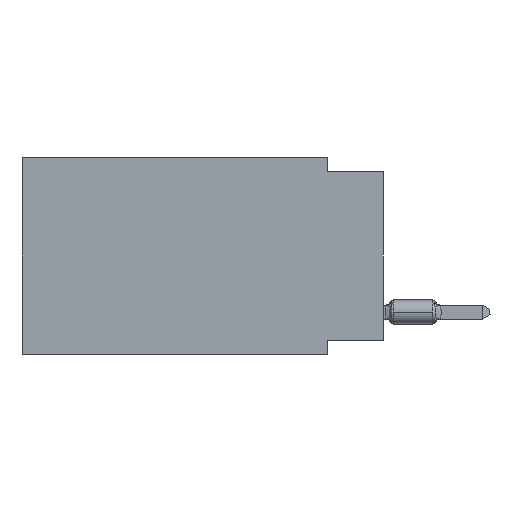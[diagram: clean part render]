
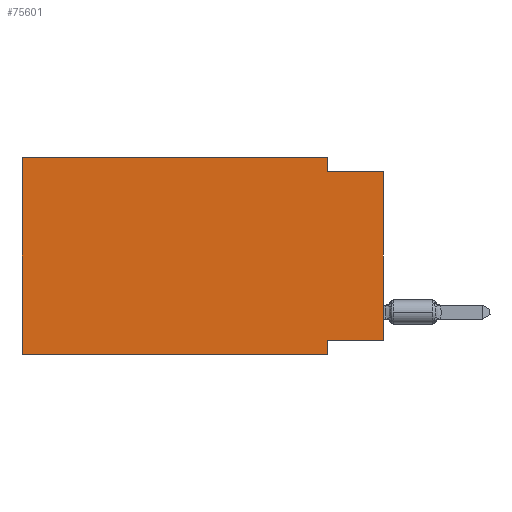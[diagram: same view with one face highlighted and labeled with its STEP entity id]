
A CAD part, left-side view. The second image highlights one B-rep face of the part: STEP entity #75601.
In plain terms, the highlighted planar face has unit normal (-1, 0, 0).
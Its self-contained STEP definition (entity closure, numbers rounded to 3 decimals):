
#530 = ORIENTED_EDGE ( 'NONE', *, *, #30145, .F. ) ;
#907 = DIRECTION ( 'NONE',  ( 1., 0., 0. ) ) ;
#2141 = VERTEX_POINT ( 'NONE', #28558 ) ;
#4248 = EDGE_CURVE ( 'NONE', #70597, #76790, #23157, .T. ) ;
#8941 = DIRECTION ( 'NONE',  ( 0., 0., -1. ) ) ;
#9344 = VECTOR ( 'NONE', #46747, 1000. ) ;
#9531 = DIRECTION ( 'NONE',  ( 0., -1., 0. ) ) ;
#12364 = CARTESIAN_POINT ( 'NONE',  ( 0., 2.54, 0. ) ) ;
#13084 = VECTOR ( 'NONE', #8941, 1000. ) ;
#14461 = EDGE_CURVE ( 'NONE', #28388, #40934, #30139, .T. ) ;
#15608 = CARTESIAN_POINT ( 'NONE',  ( 0., 16.383, -8.89 ) ) ;
#16246 = CARTESIAN_POINT ( 'NONE',  ( 0., 2.54, -0.635 ) ) ;
#17702 = ORIENTED_EDGE ( 'NONE', *, *, #14461, .F. ) ;
#20194 = CARTESIAN_POINT ( 'NONE',  ( 0., 2.54, -8.89 ) ) ;
#22602 = CARTESIAN_POINT ( 'NONE',  ( 0., 2.54, -8.89 ) ) ;
#22701 = CARTESIAN_POINT ( 'NONE',  ( 0., 0., -8.255 ) ) ;
#23157 = LINE ( 'NONE', #22701, #66028 ) ;
#23706 = DIRECTION ( 'NONE',  ( 0., 0., -1. ) ) ;
#26756 = DIRECTION ( 'NONE',  ( 0., 0., 1. ) ) ;
#28388 = VERTEX_POINT ( 'NONE', #46387 ) ;
#28558 = CARTESIAN_POINT ( 'NONE',  ( 0., 0., -0.635 ) ) ;
#30139 = LINE ( 'NONE', #65979, #54158 ) ;
#30145 = EDGE_CURVE ( 'NONE', #76790, #88114, #34155, .T. ) ;
#31007 = ORIENTED_EDGE ( 'NONE', *, *, #42371, .T. ) ;
#32056 = CARTESIAN_POINT ( 'NONE',  ( 0., 0., 0. ) ) ;
#32632 = CARTESIAN_POINT ( 'NONE',  ( 0., 0., -0.635 ) ) ;
#33211 = CARTESIAN_POINT ( 'NONE',  ( 0., 2.54, -8.255 ) ) ;
#34155 = LINE ( 'NONE', #20194, #9344 ) ;
#35707 = AXIS2_PLACEMENT_3D ( 'NONE', #37231, #907, #23706 ) ;
#37231 = CARTESIAN_POINT ( 'NONE',  ( 0., 16.383, 0. ) ) ;
#37342 = LINE ( 'NONE', #63911, #13084 ) ;
#37381 = VERTEX_POINT ( 'NONE', #88605 ) ;
#38380 = LINE ( 'NONE', #15608, #46004 ) ;
#38705 = DIRECTION ( 'NONE',  ( 0., -1., 0. ) ) ;
#40934 = VERTEX_POINT ( 'NONE', #12364 ) ;
#42003 = ORIENTED_EDGE ( 'NONE', *, *, #89813, .F. ) ;
#42371 = EDGE_CURVE ( 'NONE', #37381, #88114, #38380, .T. ) ;
#45304 = EDGE_LOOP ( 'NONE', ( #83882, #42003, #84473, #17702, #55617, #31007, #530, #53181 ) ) ;
#46004 = VECTOR ( 'NONE', #9531, 1000. ) ;
#46387 = CARTESIAN_POINT ( 'NONE',  ( 0., 16.383, 0. ) ) ;
#46747 = DIRECTION ( 'NONE',  ( 0., 0., -1. ) ) ;
#47416 = EDGE_CURVE ( 'NONE', #40934, #60084, #37342, .T. ) ;
#51959 = EDGE_CURVE ( 'NONE', #70597, #2141, #88806, .T. ) ;
#53181 = ORIENTED_EDGE ( 'NONE', *, *, #4248, .F. ) ;
#54158 = VECTOR ( 'NONE', #73867, 1000. ) ;
#55617 = ORIENTED_EDGE ( 'NONE', *, *, #58291, .F. ) ;
#58291 = EDGE_CURVE ( 'NONE', #37381, #28388, #89144, .T. ) ;
#60084 = VERTEX_POINT ( 'NONE', #16246 ) ;
#62134 = CARTESIAN_POINT ( 'NONE',  ( 0., 16.383, 0. ) ) ;
#63911 = CARTESIAN_POINT ( 'NONE',  ( 0., 2.54, 0. ) ) ;
#65979 = CARTESIAN_POINT ( 'NONE',  ( 0., 16.383, 0. ) ) ;
#66028 = VECTOR ( 'NONE', #72057, 1000. ) ;
#66406 = VECTOR ( 'NONE', #26756, 1000. ) ;
#70597 = VERTEX_POINT ( 'NONE', #74534 ) ;
#72057 = DIRECTION ( 'NONE',  ( 0., 1., 0. ) ) ;
#73509 = DIRECTION ( 'NONE',  ( 0., 0., 1. ) ) ;
#73867 = DIRECTION ( 'NONE',  ( 0., -1., 0. ) ) ;
#74534 = CARTESIAN_POINT ( 'NONE',  ( 0., 0., -8.255 ) ) ;
#75601 = ADVANCED_FACE ( 'NONE', ( #86100 ), #79589, .F. ) ;
#76790 = VERTEX_POINT ( 'NONE', #33211 ) ;
#79589 = PLANE ( 'NONE',  #35707 ) ;
#81663 = VECTOR ( 'NONE', #38705, 1000. ) ;
#83882 = ORIENTED_EDGE ( 'NONE', *, *, #51959, .T. ) ;
#84272 = VECTOR ( 'NONE', #73509, 1000. ) ;
#84473 = ORIENTED_EDGE ( 'NONE', *, *, #47416, .F. ) ;
#86100 = FACE_OUTER_BOUND ( 'NONE', #45304, .T. ) ;
#88114 = VERTEX_POINT ( 'NONE', #22602 ) ;
#88605 = CARTESIAN_POINT ( 'NONE',  ( 0., 16.383, -8.89 ) ) ;
#88806 = LINE ( 'NONE', #32056, #84272 ) ;
#88935 = LINE ( 'NONE', #32632, #81663 ) ;
#89144 = LINE ( 'NONE', #62134, #66406 ) ;
#89813 = EDGE_CURVE ( 'NONE', #60084, #2141, #88935, .T. ) ;
